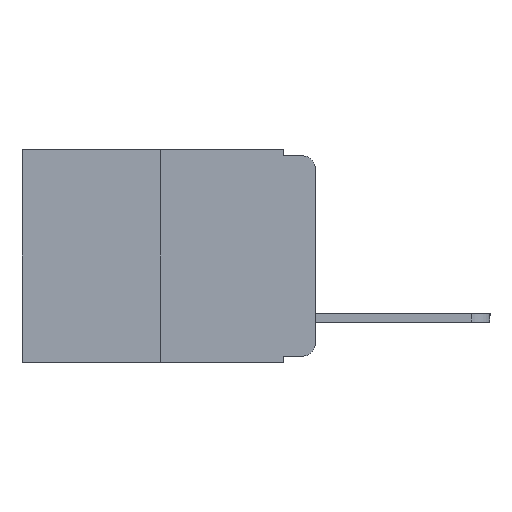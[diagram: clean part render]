
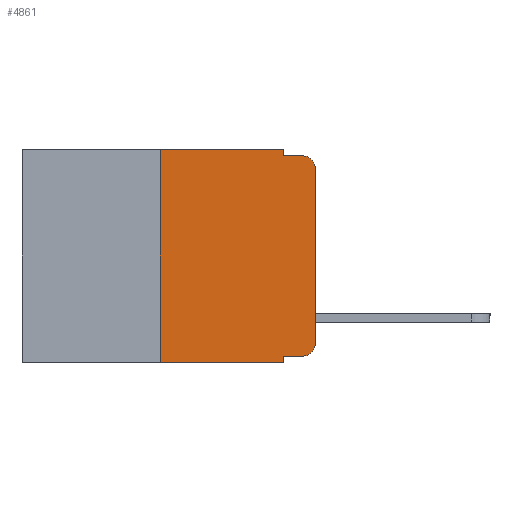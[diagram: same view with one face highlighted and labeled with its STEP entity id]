
A CAD part, left-side view. The second image highlights one B-rep face of the part: STEP entity #4861.
In plain terms, the highlighted planar face has unit normal (-1, 0, 0).
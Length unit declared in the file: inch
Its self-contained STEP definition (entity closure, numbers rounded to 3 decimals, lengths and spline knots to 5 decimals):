
#313 = CARTESIAN_POINT ( 'NONE',  ( 0., 0.02, -0.313 ) ) ;
#392 = VECTOR ( 'NONE', #3515, 39.37008 ) ;
#724 = LINE ( 'NONE', #11874, #392 ) ;
#1157 = CARTESIAN_POINT ( 'NONE',  ( 0., 0.02, -0.03 ) ) ;
#1244 = EDGE_CURVE ( 'NONE', #3136, #4980, #6507, .T. ) ;
#1404 = CARTESIAN_POINT ( 'NONE',  ( 0., 0.02, -0.333 ) ) ;
#1410 = CARTESIAN_POINT ( 'NONE',  ( 0., 0.25, 0. ) ) ;
#1413 = DIRECTION ( 'NONE',  ( 0., 0., -1. ) ) ;
#1788 = VECTOR ( 'NONE', #2096, 39.37008 ) ;
#2036 = ORIENTED_EDGE ( 'NONE', *, *, #7279, .T. ) ;
#2054 = ORIENTED_EDGE ( 'NONE', *, *, #6007, .T. ) ;
#2096 = DIRECTION ( 'NONE',  ( 0., 0., -1. ) ) ;
#2114 = ORIENTED_EDGE ( 'NONE', *, *, #4032, .F. ) ;
#2250 = DIRECTION ( 'NONE',  ( 0., 0., -1. ) ) ;
#2272 = CARTESIAN_POINT ( 'NONE',  ( 0., 0.473, -0.343 ) ) ;
#2452 = VECTOR ( 'NONE', #10808, 39.37008 ) ;
#2677 = EDGE_CURVE ( 'NONE', #6242, #4185, #4465, .T. ) ;
#2893 = ORIENTED_EDGE ( 'NONE', *, *, #12338, .F. ) ;
#3041 = ORIENTED_EDGE ( 'NONE', *, *, #11056, .T. ) ;
#3136 = VERTEX_POINT ( 'NONE', #9451 ) ;
#3143 = VERTEX_POINT ( 'NONE', #10366 ) ;
#3180 = VERTEX_POINT ( 'NONE', #8638 ) ;
#3266 = ORIENTED_EDGE ( 'NONE', *, *, #2677, .F. ) ;
#3515 = DIRECTION ( 'NONE',  ( 0., 0., -1. ) ) ;
#3596 = ORIENTED_EDGE ( 'NONE', *, *, #11119, .T. ) ;
#3610 = CARTESIAN_POINT ( 'NONE',  ( 0., 0.051, 0. ) ) ;
#3665 = ORIENTED_EDGE ( 'NONE', *, *, #9352, .T. ) ;
#4026 = CARTESIAN_POINT ( 'NONE',  ( 0., 0., -0.03 ) ) ;
#4032 = EDGE_CURVE ( 'NONE', #4185, #3143, #7419, .T. ) ;
#4167 = VECTOR ( 'NONE', #8229, 39.37008 ) ;
#4185 = VERTEX_POINT ( 'NONE', #7186 ) ;
#4465 = LINE ( 'NONE', #5063, #1788 ) ;
#4832 = ORIENTED_EDGE ( 'NONE', *, *, #1244, .F. ) ;
#4861 = ADVANCED_FACE ( 'NONE', ( #6056 ), #5286, .F. ) ;
#4980 = VERTEX_POINT ( 'NONE', #1410 ) ;
#5063 = CARTESIAN_POINT ( 'NONE',  ( 0., 0.051, 0. ) ) ;
#5072 = CARTESIAN_POINT ( 'NONE',  ( 0., 0.051, -0.01 ) ) ;
#5095 = LINE ( 'NONE', #2272, #2452 ) ;
#5170 = ORIENTED_EDGE ( 'NONE', *, *, #9824, .F. ) ;
#5188 = CARTESIAN_POINT ( 'NONE',  ( 0., 0., 0. ) ) ;
#5216 = VECTOR ( 'NONE', #9004, 39.37008 ) ;
#5286 = PLANE ( 'NONE',  #10809 ) ;
#5456 = CARTESIAN_POINT ( 'NONE',  ( 0., 0.25, 0. ) ) ;
#5586 = AXIS2_PLACEMENT_3D ( 'NONE', #1157, #8083, #2250 ) ;
#5859 = VERTEX_POINT ( 'NONE', #6039 ) ;
#6007 = EDGE_CURVE ( 'NONE', #11371, #3143, #7803, .T. ) ;
#6039 = CARTESIAN_POINT ( 'NONE',  ( 0., 0., -0.313 ) ) ;
#6056 = FACE_OUTER_BOUND ( 'NONE', #7401, .T. ) ;
#6168 = DIRECTION ( 'NONE',  ( 0., -1., 0. ) ) ;
#6201 = VECTOR ( 'NONE', #6686, 39.37008 ) ;
#6242 = VERTEX_POINT ( 'NONE', #3610 ) ;
#6301 = DIRECTION ( 'NONE',  ( 0., 0., -1. ) ) ;
#6507 = LINE ( 'NONE', #5456, #6201 ) ;
#6686 = DIRECTION ( 'NONE',  ( 0., 0., 1. ) ) ;
#6770 = LINE ( 'NONE', #11776, #4167 ) ;
#7186 = CARTESIAN_POINT ( 'NONE',  ( 0., 0.051, -0.01 ) ) ;
#7279 = EDGE_CURVE ( 'NONE', #5859, #11371, #8347, .T. ) ;
#7387 = DIRECTION ( 'NONE',  ( -1., 0., 0. ) ) ;
#7401 = EDGE_LOOP ( 'NONE', ( #2036, #2054, #2114, #3266, #5170, #4832, #3041, #2893, #3596, #3665 ) ) ;
#7407 = VERTEX_POINT ( 'NONE', #8265 ) ;
#7419 = LINE ( 'NONE', #5072, #7712 ) ;
#7479 = VERTEX_POINT ( 'NONE', #1404 ) ;
#7712 = VECTOR ( 'NONE', #11511, 39.37008 ) ;
#7803 = CIRCLE ( 'NONE', #5586, 0.02 ) ;
#7971 = VECTOR ( 'NONE', #6168, 39.37008 ) ;
#8083 = DIRECTION ( 'NONE',  ( -1., 0., 0. ) ) ;
#8229 = DIRECTION ( 'NONE',  ( 0., -1., 0. ) ) ;
#8265 = CARTESIAN_POINT ( 'NONE',  ( 0., 0.051, -0.343 ) ) ;
#8347 = LINE ( 'NONE', #5188, #5216 ) ;
#8638 = CARTESIAN_POINT ( 'NONE',  ( 0., 0.051, -0.333 ) ) ;
#9004 = DIRECTION ( 'NONE',  ( 0., 0., 1. ) ) ;
#9081 = CARTESIAN_POINT ( 'NONE',  ( 0., 0.473, 0. ) ) ;
#9352 = EDGE_CURVE ( 'NONE', #7479, #5859, #11086, .T. ) ;
#9451 = CARTESIAN_POINT ( 'NONE',  ( 0., 0.25, -0.343 ) ) ;
#9824 = EDGE_CURVE ( 'NONE', #4980, #6242, #10381, .T. ) ;
#10366 = CARTESIAN_POINT ( 'NONE',  ( 0., 0.02, -0.01 ) ) ;
#10381 = LINE ( 'NONE', #10726, #7971 ) ;
#10726 = CARTESIAN_POINT ( 'NONE',  ( 0., 0.473, 0. ) ) ;
#10808 = DIRECTION ( 'NONE',  ( 0., -1., 0. ) ) ;
#10809 = AXIS2_PLACEMENT_3D ( 'NONE', #9081, #11732, #6301 ) ;
#11056 = EDGE_CURVE ( 'NONE', #3136, #7407, #5095, .T. ) ;
#11086 = CIRCLE ( 'NONE', #12271, 0.02 ) ;
#11119 = EDGE_CURVE ( 'NONE', #3180, #7479, #6770, .T. ) ;
#11371 = VERTEX_POINT ( 'NONE', #4026 ) ;
#11511 = DIRECTION ( 'NONE',  ( 0., -1., 0. ) ) ;
#11732 = DIRECTION ( 'NONE',  ( 1., 0., 0. ) ) ;
#11776 = CARTESIAN_POINT ( 'NONE',  ( 0., 0.051, -0.333 ) ) ;
#11874 = CARTESIAN_POINT ( 'NONE',  ( 0., 0.051, 0. ) ) ;
#12271 = AXIS2_PLACEMENT_3D ( 'NONE', #313, #7387, #1413 ) ;
#12338 = EDGE_CURVE ( 'NONE', #3180, #7407, #724, .T. ) ;
